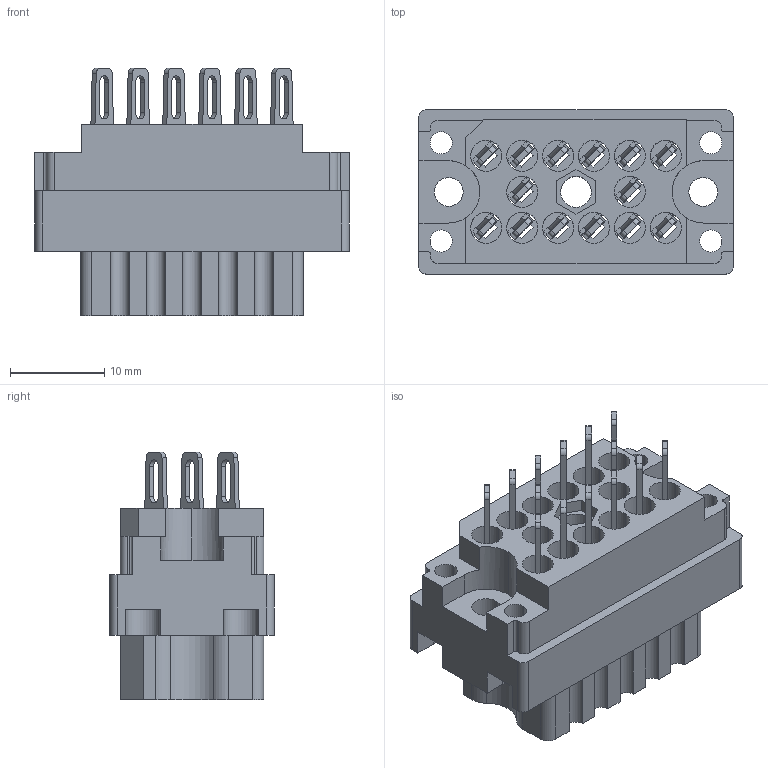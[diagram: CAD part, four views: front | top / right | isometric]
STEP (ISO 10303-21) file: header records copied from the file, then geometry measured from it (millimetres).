
FILE_DESCRIPTION (( 'STEP AP203' ), '1' );
FILE_NAME ('519-014-500-400.STEP', '2020-09-09T17:44:12', ( '' ), ( '' ), 'SwSTEP 2.0', 'SolidWorks 2020', '' );
FILE_SCHEMA (( 'CONFIG_CONTROL_DESIGN' ));
Length unit declared in the file: inch
Products named in the file (3): 519 Receptacle Insulator_014; 519-014-500-400; 516-292-001_500 Contact
Assembly tree (15 placements, depth 2):
  519-014-500-400
    519 Receptacle Insulator_014
    516-292-001_500 Contact  x14
Bounding box: 33.32 x 17.42 x 26.21 mm (x, y, z)
Volume: 6581.7 mm3; surface area: 9421.6 mm2
Topology: 15 solids, 15 shells, 1541 faces, 4471 edges, 2970 vertices
Faces by surface type: plane 925, cylinder 530, bspline 84, cone 2
Entity records: 19297 total; most frequent: CARTESIAN_POINT 3539, ORIENTED_EDGE 3222, DIRECTION 3117, EDGE_CURVE 1611, LINE 1167, VECTOR 1167, VERTEX_POINT 1072, AXIS2_PLACEMENT_3D 975
